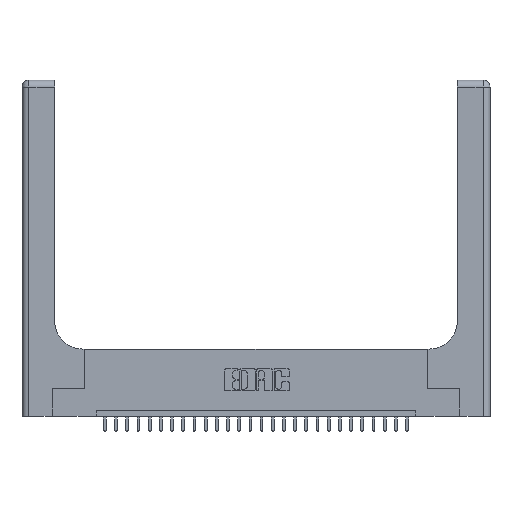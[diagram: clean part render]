
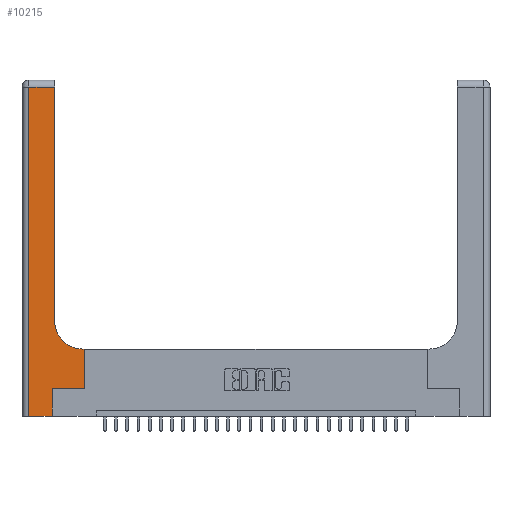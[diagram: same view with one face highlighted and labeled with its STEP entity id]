
A CAD part, top view. The second image highlights one B-rep face of the part: STEP entity #10215.
In plain terms, the highlighted planar face has unit normal (0, 0, 1).
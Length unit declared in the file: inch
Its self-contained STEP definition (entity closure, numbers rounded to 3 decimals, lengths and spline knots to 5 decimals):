
#192 = VECTOR ( 'NONE', #25333, 39.37008 ) ;
#199 = EDGE_CURVE ( 'NONE', #3936, #11803, #733, .T. ) ;
#338 = VERTEX_POINT ( 'NONE', #23251 ) ;
#733 = LINE ( 'NONE', #14185, #11612 ) ;
#798 = VECTOR ( 'NONE', #11587, 39.37008 ) ;
#972 = EDGE_LOOP ( 'NONE', ( #19680, #17551, #7965, #28010, #9910, #26510, #18110, #5407, #9513 ) ) ;
#1002 = LINE ( 'NONE', #27195, #16354 ) ;
#1154 = DIRECTION ( 'NONE',  ( -1., 0., 0. ) ) ;
#1870 = CARTESIAN_POINT ( 'NONE',  ( 0.269, 0.25, 0.37 ) ) ;
#2369 = EDGE_CURVE ( 'NONE', #22509, #12571, #18314, .T. ) ;
#2385 = VECTOR ( 'NONE', #8149, 39.37008 ) ;
#2396 = VERTEX_POINT ( 'NONE', #5121 ) ;
#2700 = CARTESIAN_POINT ( 'NONE',  ( 0.269, 0., 0.37 ) ) ;
#2930 = LINE ( 'NONE', #20681, #3627 ) ;
#3604 = EDGE_CURVE ( 'NONE', #338, #13087, #21627, .T. ) ;
#3627 = VECTOR ( 'NONE', #18325, 39.37008 ) ;
#3682 = EDGE_CURVE ( 'NONE', #12571, #11295, #4286, .T. ) ;
#3936 = VERTEX_POINT ( 'NONE', #22702 ) ;
#4286 = LINE ( 'NONE', #18972, #192 ) ;
#4490 = AXIS2_PLACEMENT_3D ( 'NONE', #10660, #25585, #12835 ) ;
#4656 = CARTESIAN_POINT ( 'NONE',  ( 0.5585, 0.6, 0.37 ) ) ;
#5121 = CARTESIAN_POINT ( 'NONE',  ( 0.269, 0.25, 0.37 ) ) ;
#5340 = CARTESIAN_POINT ( 'NONE',  ( 0.5415, 0.6, 0.37 ) ) ;
#5407 = ORIENTED_EDGE ( 'NONE', *, *, #16318, .T. ) ;
#6986 = CARTESIAN_POINT ( 'NONE',  ( 0.269, 0., 0.37 ) ) ;
#7357 = AXIS2_PLACEMENT_3D ( 'NONE', #8206, #25269, #14446 ) ;
#7965 = ORIENTED_EDGE ( 'NONE', *, *, #3604, .T. ) ;
#8149 = DIRECTION ( 'NONE',  ( 1., 0., 0. ) ) ;
#8206 = CARTESIAN_POINT ( 'NONE',  ( 0., 3., 0.37 ) ) ;
#8303 = CARTESIAN_POINT ( 'NONE',  ( 0.2915, 0.85, 0.37 ) ) ;
#9513 = ORIENTED_EDGE ( 'NONE', *, *, #2369, .T. ) ;
#9910 = ORIENTED_EDGE ( 'NONE', *, *, #25336, .T. ) ;
#10215 = ADVANCED_FACE ( 'NONE', ( #23309 ), #12446, .F. ) ;
#10660 = CARTESIAN_POINT ( 'NONE',  ( 0.5415, 0.85, 0.37 ) ) ;
#11230 = LINE ( 'NONE', #6986, #25189 ) ;
#11295 = VERTEX_POINT ( 'NONE', #23351 ) ;
#11587 = DIRECTION ( 'NONE',  ( 1., 0., 0. ) ) ;
#11612 = VECTOR ( 'NONE', #16413, 39.37008 ) ;
#11803 = VERTEX_POINT ( 'NONE', #4656 ) ;
#12446 = PLANE ( 'NONE',  #7357 ) ;
#12571 = VERTEX_POINT ( 'NONE', #8303 ) ;
#12835 = DIRECTION ( 'NONE',  ( 1., 0., 0. ) ) ;
#13087 = VERTEX_POINT ( 'NONE', #18954 ) ;
#13134 = VECTOR ( 'NONE', #27816, 39.37008 ) ;
#14185 = CARTESIAN_POINT ( 'NONE',  ( 0.5585, 0.25, 0.37 ) ) ;
#14446 = DIRECTION ( 'NONE',  ( -1., 0., 0. ) ) ;
#15376 = CARTESIAN_POINT ( 'NONE',  ( 0., 0., 0.37 ) ) ;
#16318 = EDGE_CURVE ( 'NONE', #11803, #22509, #1002, .T. ) ;
#16354 = VECTOR ( 'NONE', #1154, 39.37008 ) ;
#16413 = DIRECTION ( 'NONE',  ( 0., 1., 0. ) ) ;
#17551 = ORIENTED_EDGE ( 'NONE', *, *, #18174, .T. ) ;
#18110 = ORIENTED_EDGE ( 'NONE', *, *, #199, .T. ) ;
#18174 = EDGE_CURVE ( 'NONE', #11295, #338, #2930, .T. ) ;
#18314 = CIRCLE ( 'NONE', #4490, 0.25 ) ;
#18325 = DIRECTION ( 'NONE',  ( -1., 0., 0. ) ) ;
#18954 = CARTESIAN_POINT ( 'NONE',  ( 0.06, 0., 0.37 ) ) ;
#18972 = CARTESIAN_POINT ( 'NONE',  ( 0.2915, 3., 0.37 ) ) ;
#19680 = ORIENTED_EDGE ( 'NONE', *, *, #3682, .T. ) ;
#20681 = CARTESIAN_POINT ( 'NONE',  ( 0., 2.94, 0.37 ) ) ;
#21237 = LINE ( 'NONE', #15376, #798 ) ;
#21627 = LINE ( 'NONE', #22594, #13134 ) ;
#21739 = LINE ( 'NONE', #1870, #2385 ) ;
#22152 = DIRECTION ( 'NONE',  ( 0., 1., 0. ) ) ;
#22509 = VERTEX_POINT ( 'NONE', #5340 ) ;
#22594 = CARTESIAN_POINT ( 'NONE',  ( 0.06, 3., 0.37 ) ) ;
#22702 = CARTESIAN_POINT ( 'NONE',  ( 0.5585, 0.25, 0.37 ) ) ;
#23092 = EDGE_CURVE ( 'NONE', #13087, #27447, #21237, .T. ) ;
#23251 = CARTESIAN_POINT ( 'NONE',  ( 0.06, 2.94, 0.37 ) ) ;
#23309 = FACE_OUTER_BOUND ( 'NONE', #972, .T. ) ;
#23351 = CARTESIAN_POINT ( 'NONE',  ( 0.2915, 2.94, 0.37 ) ) ;
#25189 = VECTOR ( 'NONE', #22152, 39.37008 ) ;
#25269 = DIRECTION ( 'NONE',  ( 0., 0., -1. ) ) ;
#25333 = DIRECTION ( 'NONE',  ( 0., 1., 0. ) ) ;
#25336 = EDGE_CURVE ( 'NONE', #27447, #2396, #11230, .T. ) ;
#25585 = DIRECTION ( 'NONE',  ( 0., 0., -1. ) ) ;
#25740 = EDGE_CURVE ( 'NONE', #2396, #3936, #21739, .T. ) ;
#26510 = ORIENTED_EDGE ( 'NONE', *, *, #25740, .T. ) ;
#27195 = CARTESIAN_POINT ( 'NONE',  ( 0.2915, 0.6, 0.37 ) ) ;
#27447 = VERTEX_POINT ( 'NONE', #2700 ) ;
#27816 = DIRECTION ( 'NONE',  ( 0., -1., 0. ) ) ;
#28010 = ORIENTED_EDGE ( 'NONE', *, *, #23092, .T. ) ;
